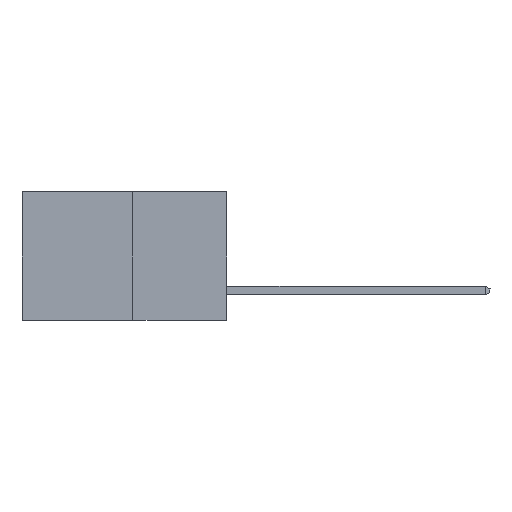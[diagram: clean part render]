
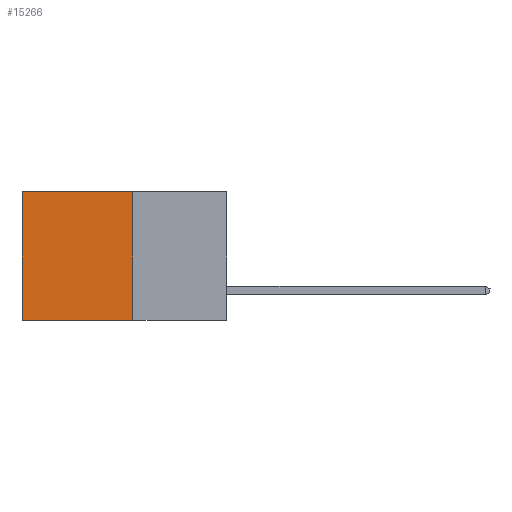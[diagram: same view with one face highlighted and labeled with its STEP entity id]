
A CAD part, left-side view. The second image highlights one B-rep face of the part: STEP entity #15266.
In plain terms, the highlighted planar face has unit normal (-1, 0, 0).
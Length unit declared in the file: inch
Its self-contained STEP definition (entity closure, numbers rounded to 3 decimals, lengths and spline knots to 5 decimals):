
#16 = VERTEX_POINT ( 'NONE', #12904 ) ;
#1061 = EDGE_CURVE ( 'NONE', #5390, #8848, #1355, .T. ) ;
#1117 = EDGE_CURVE ( 'NONE', #15230, #16, #7186, .T. ) ;
#1355 = LINE ( 'NONE', #4098, #7987 ) ;
#1370 = EDGE_LOOP ( 'NONE', ( #6623, #7344, #7639, #7936 ) ) ;
#1447 = CARTESIAN_POINT ( 'NONE',  ( 0.277, 0.59, -0.37 ) ) ;
#1687 = DIRECTION ( 'NONE',  ( 0., 0., -1. ) ) ;
#3532 = FACE_OUTER_BOUND ( 'NONE', #1370, .T. ) ;
#4098 = CARTESIAN_POINT ( 'NONE',  ( 0.277, 0.27, -0.37 ) ) ;
#4135 = EDGE_CURVE ( 'NONE', #5390, #15230, #7622, .T. ) ;
#4174 = CARTESIAN_POINT ( 'NONE',  ( 0.277, 0.27, -0.37 ) ) ;
#5196 = EDGE_CURVE ( 'NONE', #8848, #16, #10749, .T. ) ;
#5390 = VERTEX_POINT ( 'NONE', #8509 ) ;
#6623 = ORIENTED_EDGE ( 'NONE', *, *, #1117, .T. ) ;
#6787 = VECTOR ( 'NONE', #11360, 39.37008 ) ;
#7186 = LINE ( 'NONE', #1447, #6787 ) ;
#7344 = ORIENTED_EDGE ( 'NONE', *, *, #5196, .F. ) ;
#7622 = LINE ( 'NONE', #8596, #13267 ) ;
#7639 = ORIENTED_EDGE ( 'NONE', *, *, #1061, .F. ) ;
#7936 = ORIENTED_EDGE ( 'NONE', *, *, #4135, .T. ) ;
#7987 = VECTOR ( 'NONE', #13489, 39.37008 ) ;
#8239 = CARTESIAN_POINT ( 'NONE',  ( 0.277, 0.27, -0.37 ) ) ;
#8509 = CARTESIAN_POINT ( 'NONE',  ( 0.277, 0.27, 0. ) ) ;
#8579 = DIRECTION ( 'NONE',  ( 0., 1., 0. ) ) ;
#8596 = CARTESIAN_POINT ( 'NONE',  ( 0.277, 0.27, 0. ) ) ;
#8848 = VERTEX_POINT ( 'NONE', #4174 ) ;
#9369 = CARTESIAN_POINT ( 'NONE',  ( 0.277, 0.59, 0. ) ) ;
#9467 = DIRECTION ( 'NONE',  ( 1., 0., 0. ) ) ;
#10286 = DIRECTION ( 'NONE',  ( 0., 1., 0. ) ) ;
#10305 = CARTESIAN_POINT ( 'NONE',  ( 0.277, 0.27, -0.37 ) ) ;
#10749 = LINE ( 'NONE', #10305, #16131 ) ;
#11360 = DIRECTION ( 'NONE',  ( 0., 0., -1. ) ) ;
#12904 = CARTESIAN_POINT ( 'NONE',  ( 0.277, 0.59, -0.37 ) ) ;
#12985 = PLANE ( 'NONE',  #13084 ) ;
#13084 = AXIS2_PLACEMENT_3D ( 'NONE', #8239, #9467, #1687 ) ;
#13267 = VECTOR ( 'NONE', #8579, 39.37008 ) ;
#13489 = DIRECTION ( 'NONE',  ( 0., 0., -1. ) ) ;
#15230 = VERTEX_POINT ( 'NONE', #9369 ) ;
#15266 = ADVANCED_FACE ( 'NONE', ( #3532 ), #12985, .F. ) ;
#16131 = VECTOR ( 'NONE', #10286, 39.37008 ) ;
